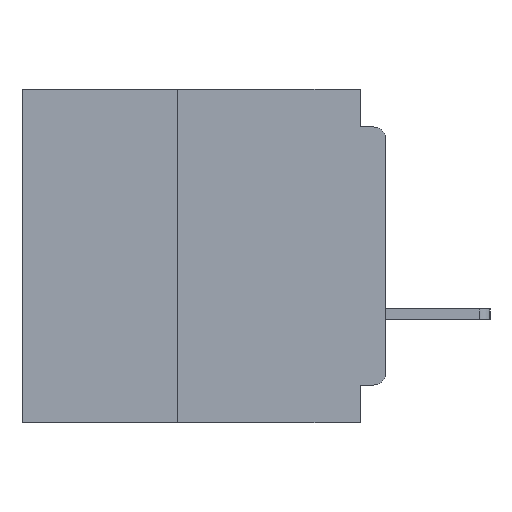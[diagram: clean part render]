
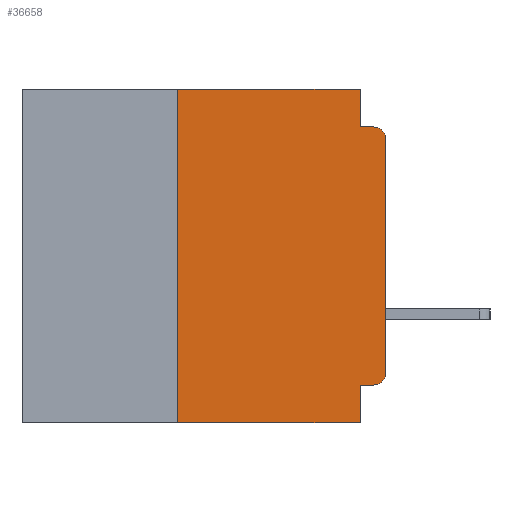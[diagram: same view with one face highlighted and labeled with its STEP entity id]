
A CAD part, left-side view. The second image highlights one B-rep face of the part: STEP entity #36658.
In plain terms, the highlighted planar face has unit normal (-1, 0, 0).
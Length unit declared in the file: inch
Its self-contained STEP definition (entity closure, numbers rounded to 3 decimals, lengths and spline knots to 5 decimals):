
#235 = LINE ( 'NONE', #12220, #7290 ) ;
#486 = CARTESIAN_POINT ( 'NONE',  ( 0., 0.031, -0.355 ) ) ;
#525 = CARTESIAN_POINT ( 'NONE',  ( 0., 0.015, -0.34 ) ) ;
#535 = CARTESIAN_POINT ( 'NONE',  ( 0., 0.031, -0.045 ) ) ;
#757 = CARTESIAN_POINT ( 'NONE',  ( 0., 0.015, -0.045 ) ) ;
#820 = CARTESIAN_POINT ( 'NONE',  ( 0., 0.031, 0. ) ) ;
#1803 = CARTESIAN_POINT ( 'NONE',  ( 0., 0., 0. ) ) ;
#2107 = VERTEX_POINT ( 'NONE', #33427 ) ;
#2224 = VECTOR ( 'NONE', #35279, 39.37008 ) ;
#2244 = LINE ( 'NONE', #20247, #25283 ) ;
#2639 = LINE ( 'NONE', #1803, #31778 ) ;
#3596 = DIRECTION ( 'NONE',  ( 0., 0., -1. ) ) ;
#3940 = ORIENTED_EDGE ( 'NONE', *, *, #15045, .T. ) ;
#4362 = CARTESIAN_POINT ( 'NONE',  ( 0., 0.031, -0.4 ) ) ;
#4689 = VERTEX_POINT ( 'NONE', #24451 ) ;
#5328 = VERTEX_POINT ( 'NONE', #535 ) ;
#5801 = ORIENTED_EDGE ( 'NONE', *, *, #6222, .F. ) ;
#6222 = EDGE_CURVE ( 'NONE', #5328, #37976, #6954, .T. ) ;
#6422 = ORIENTED_EDGE ( 'NONE', *, *, #26099, .F. ) ;
#6954 = LINE ( 'NONE', #22699, #7861 ) ;
#7154 = EDGE_LOOP ( 'NONE', ( #9501, #16648, #5801, #14215, #9931, #6422, #37335, #21816, #35502, #3940 ) ) ;
#7290 = VECTOR ( 'NONE', #27218, 39.37008 ) ;
#7323 = DIRECTION ( 'NONE',  ( 0., 0., -1. ) ) ;
#7532 = CIRCLE ( 'NONE', #18706, 0.015 ) ;
#7861 = VECTOR ( 'NONE', #23524, 39.37008 ) ;
#9361 = PLANE ( 'NONE',  #31492 ) ;
#9501 = ORIENTED_EDGE ( 'NONE', *, *, #22376, .T. ) ;
#9931 = ORIENTED_EDGE ( 'NONE', *, *, #36001, .F. ) ;
#11340 = CARTESIAN_POINT ( 'NONE',  ( 0., 0.015, -0.06 ) ) ;
#12220 = CARTESIAN_POINT ( 'NONE',  ( 0., 0.25, -0.4 ) ) ;
#12635 = LINE ( 'NONE', #12956, #24881 ) ;
#12956 = CARTESIAN_POINT ( 'NONE',  ( 0., 0.031, 0. ) ) ;
#13746 = DIRECTION ( 'NONE',  ( 0., 0., 1. ) ) ;
#14215 = ORIENTED_EDGE ( 'NONE', *, *, #30147, .F. ) ;
#14367 = DIRECTION ( 'NONE',  ( 0., 0., -1. ) ) ;
#15045 = EDGE_CURVE ( 'NONE', #4689, #33275, #30017, .T. ) ;
#15468 = DIRECTION ( 'NONE',  ( 1., 0., 0. ) ) ;
#15782 = VERTEX_POINT ( 'NONE', #16024 ) ;
#16024 = CARTESIAN_POINT ( 'NONE',  ( 0., 0.25, -0.4 ) ) ;
#16648 = ORIENTED_EDGE ( 'NONE', *, *, #23121, .T. ) ;
#17407 = VERTEX_POINT ( 'NONE', #820 ) ;
#17635 = DIRECTION ( 'NONE',  ( 0., -1., 0. ) ) ;
#18063 = EDGE_CURVE ( 'NONE', #31426, #20181, #18482, .T. ) ;
#18482 = LINE ( 'NONE', #4362, #33516 ) ;
#18706 = AXIS2_PLACEMENT_3D ( 'NONE', #11340, #32398, #14367 ) ;
#20181 = VERTEX_POINT ( 'NONE', #31796 ) ;
#20247 = CARTESIAN_POINT ( 'NONE',  ( 0., 0.437, 0. ) ) ;
#21598 = DIRECTION ( 'NONE',  ( -1., 0., 0. ) ) ;
#21816 = ORIENTED_EDGE ( 'NONE', *, *, #18063, .F. ) ;
#22072 = DIRECTION ( 'NONE',  ( 0., 0., -1. ) ) ;
#22101 = EDGE_CURVE ( 'NONE', #15782, #20181, #33637, .T. ) ;
#22376 = EDGE_CURVE ( 'NONE', #33275, #2107, #2639, .T. ) ;
#22699 = CARTESIAN_POINT ( 'NONE',  ( 0., 0., -0.045 ) ) ;
#23121 = EDGE_CURVE ( 'NONE', #2107, #37976, #7532, .T. ) ;
#23237 = DIRECTION ( 'NONE',  ( 0., -1., 0. ) ) ;
#23288 = CARTESIAN_POINT ( 'NONE',  ( 0., 0., -0.355 ) ) ;
#23524 = DIRECTION ( 'NONE',  ( 0., -1., 0. ) ) ;
#23656 = CARTESIAN_POINT ( 'NONE',  ( 0., 0.437, -0.4 ) ) ;
#24451 = CARTESIAN_POINT ( 'NONE',  ( 0., 0.015, -0.355 ) ) ;
#24686 = VECTOR ( 'NONE', #17635, 39.37008 ) ;
#24881 = VECTOR ( 'NONE', #22072, 39.37008 ) ;
#25283 = VECTOR ( 'NONE', #23237, 39.37008 ) ;
#26099 = EDGE_CURVE ( 'NONE', #15782, #31127, #235, .T. ) ;
#26208 = LINE ( 'NONE', #23288, #2224 ) ;
#27218 = DIRECTION ( 'NONE',  ( 0., 0., 1. ) ) ;
#27308 = CARTESIAN_POINT ( 'NONE',  ( 0., 0., -0.34 ) ) ;
#30017 = CIRCLE ( 'NONE', #30778, 0.015 ) ;
#30147 = EDGE_CURVE ( 'NONE', #17407, #5328, #12635, .T. ) ;
#30778 = AXIS2_PLACEMENT_3D ( 'NONE', #525, #21598, #3596 ) ;
#31127 = VERTEX_POINT ( 'NONE', #35152 ) ;
#31159 = EDGE_CURVE ( 'NONE', #4689, #31426, #26208, .T. ) ;
#31426 = VERTEX_POINT ( 'NONE', #486 ) ;
#31492 = AXIS2_PLACEMENT_3D ( 'NONE', #33490, #15468, #36549 ) ;
#31778 = VECTOR ( 'NONE', #13746, 39.37008 ) ;
#31796 = CARTESIAN_POINT ( 'NONE',  ( 0., 0.031, -0.4 ) ) ;
#32398 = DIRECTION ( 'NONE',  ( -1., 0., 0. ) ) ;
#33275 = VERTEX_POINT ( 'NONE', #27308 ) ;
#33427 = CARTESIAN_POINT ( 'NONE',  ( 0., 0., -0.06 ) ) ;
#33490 = CARTESIAN_POINT ( 'NONE',  ( 0., 0.437, 0. ) ) ;
#33516 = VECTOR ( 'NONE', #7323, 39.37008 ) ;
#33637 = LINE ( 'NONE', #23656, #24686 ) ;
#33709 = FACE_OUTER_BOUND ( 'NONE', #7154, .T. ) ;
#35152 = CARTESIAN_POINT ( 'NONE',  ( 0., 0.25, 0. ) ) ;
#35279 = DIRECTION ( 'NONE',  ( 0., 1., 0. ) ) ;
#35502 = ORIENTED_EDGE ( 'NONE', *, *, #31159, .F. ) ;
#36001 = EDGE_CURVE ( 'NONE', #31127, #17407, #2244, .T. ) ;
#36549 = DIRECTION ( 'NONE',  ( 0., 0., -1. ) ) ;
#36658 = ADVANCED_FACE ( 'NONE', ( #33709 ), #9361, .F. ) ;
#37335 = ORIENTED_EDGE ( 'NONE', *, *, #22101, .T. ) ;
#37976 = VERTEX_POINT ( 'NONE', #757 ) ;
